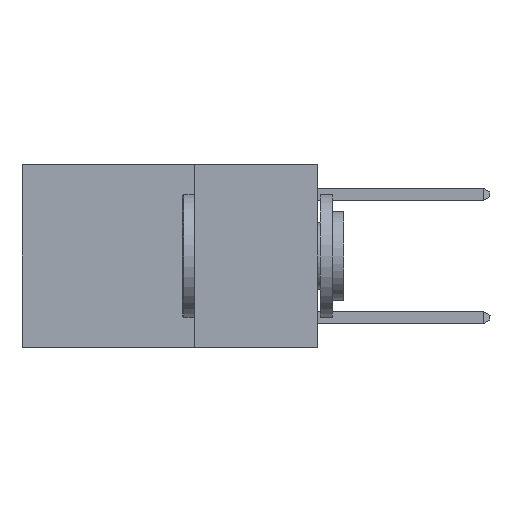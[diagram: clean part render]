
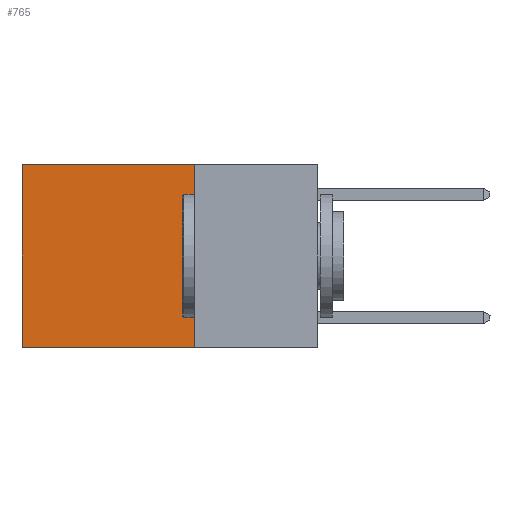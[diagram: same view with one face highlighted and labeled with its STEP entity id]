
A CAD part, left-side view. The second image highlights one B-rep face of the part: STEP entity #765.
In plain terms, the highlighted planar face has unit normal (-1, 0, 0).
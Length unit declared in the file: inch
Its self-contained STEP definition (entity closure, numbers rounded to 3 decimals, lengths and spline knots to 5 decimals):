
#395 = CARTESIAN_POINT ( 'NONE',  ( 0.2625, 0.25, -0.37 ) ) ;
#765 = ADVANCED_FACE ( 'NONE', ( #6567 ), #11141, .F. ) ;
#2455 = LINE ( 'NONE', #8793, #25761 ) ;
#3425 = VERTEX_POINT ( 'NONE', #5538 ) ;
#4099 = DIRECTION ( 'NONE',  ( 0., 1., 0. ) ) ;
#4784 = VERTEX_POINT ( 'NONE', #24973 ) ;
#5300 = CARTESIAN_POINT ( 'NONE',  ( 0.2625, 0.25, 0. ) ) ;
#5538 = CARTESIAN_POINT ( 'NONE',  ( 0.2625, 0.6, 0. ) ) ;
#5595 = LINE ( 'NONE', #12605, #28600 ) ;
#6567 = FACE_OUTER_BOUND ( 'NONE', #17663, .T. ) ;
#6694 = CARTESIAN_POINT ( 'NONE',  ( 0.2625, 0.6, 0. ) ) ;
#7180 = VECTOR ( 'NONE', #12437, 39.37008 ) ;
#8793 = CARTESIAN_POINT ( 'NONE',  ( 0.2625, 0.25, -0.37 ) ) ;
#11141 = PLANE ( 'NONE',  #17519 ) ;
#11457 = DIRECTION ( 'NONE',  ( 0., 0., -1. ) ) ;
#12437 = DIRECTION ( 'NONE',  ( 0., 0., -1. ) ) ;
#12605 = CARTESIAN_POINT ( 'NONE',  ( 0.2625, 0.25, 0. ) ) ;
#12755 = LINE ( 'NONE', #6694, #23753 ) ;
#13407 = DIRECTION ( 'NONE',  ( 1., 0., 0. ) ) ;
#14017 = ORIENTED_EDGE ( 'NONE', *, *, #18546, .F. ) ;
#14707 = ORIENTED_EDGE ( 'NONE', *, *, #21400, .T. ) ;
#15948 = CARTESIAN_POINT ( 'NONE',  ( 0.2625, 0.6, -0.37 ) ) ;
#17519 = AXIS2_PLACEMENT_3D ( 'NONE', #26480, #13407, #28593 ) ;
#17663 = EDGE_LOOP ( 'NONE', ( #24993, #14017, #25654, #14707 ) ) ;
#18546 = EDGE_CURVE ( 'NONE', #26129, #24127, #2455, .T. ) ;
#18664 = EDGE_CURVE ( 'NONE', #3425, #24127, #12755, .T. ) ;
#19980 = LINE ( 'NONE', #5300, #7180 ) ;
#21400 = EDGE_CURVE ( 'NONE', #4784, #3425, #5595, .T. ) ;
#23548 = DIRECTION ( 'NONE',  ( 0., 1., 0. ) ) ;
#23753 = VECTOR ( 'NONE', #11457, 39.37008 ) ;
#24127 = VERTEX_POINT ( 'NONE', #15948 ) ;
#24506 = EDGE_CURVE ( 'NONE', #4784, #26129, #19980, .T. ) ;
#24973 = CARTESIAN_POINT ( 'NONE',  ( 0.2625, 0.25, 0. ) ) ;
#24993 = ORIENTED_EDGE ( 'NONE', *, *, #18664, .T. ) ;
#25654 = ORIENTED_EDGE ( 'NONE', *, *, #24506, .F. ) ;
#25761 = VECTOR ( 'NONE', #4099, 39.37008 ) ;
#26129 = VERTEX_POINT ( 'NONE', #395 ) ;
#26480 = CARTESIAN_POINT ( 'NONE',  ( 0.2625, 0.25, 0. ) ) ;
#28593 = DIRECTION ( 'NONE',  ( 0., 0., -1. ) ) ;
#28600 = VECTOR ( 'NONE', #23548, 39.37008 ) ;
